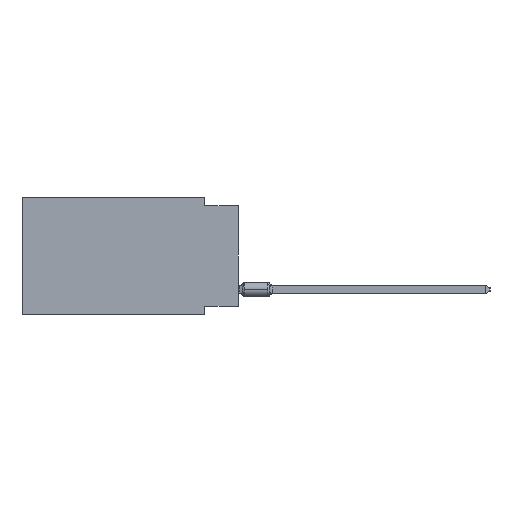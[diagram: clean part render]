
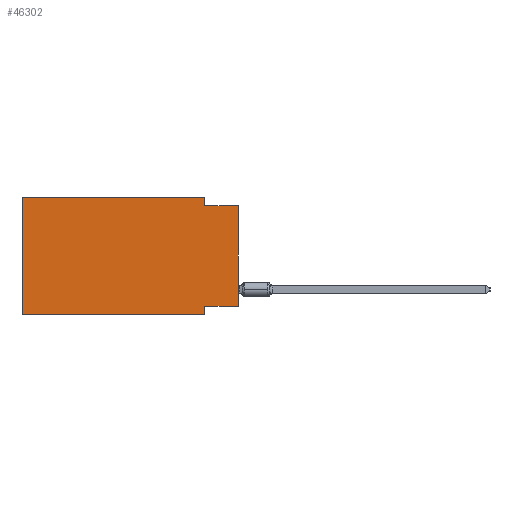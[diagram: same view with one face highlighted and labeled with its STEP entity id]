
A CAD part, left-side view. The second image highlights one B-rep face of the part: STEP entity #46302.
In plain terms, the highlighted planar face has unit normal (-1, 0, 0).
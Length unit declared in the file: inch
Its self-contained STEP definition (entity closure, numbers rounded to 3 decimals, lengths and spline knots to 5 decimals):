
#163 = DIRECTION ( 'NONE',  ( 0., -1., 0. ) ) ;
#812 = DIRECTION ( 'NONE',  ( 0., 0., -1. ) ) ;
#1198 = VECTOR ( 'NONE', #1900, 39.37008 ) ;
#1242 = ORIENTED_EDGE ( 'NONE', *, *, #15102, .F. ) ;
#1676 = ORIENTED_EDGE ( 'NONE', *, *, #29330, .T. ) ;
#1728 = DIRECTION ( 'NONE',  ( 0., -1., 0. ) ) ;
#1900 = DIRECTION ( 'NONE',  ( 0., 0., -1. ) ) ;
#2158 = LINE ( 'NONE', #32394, #14801 ) ;
#2574 = CARTESIAN_POINT ( 'NONE',  ( 0., 0., -0.025 ) ) ;
#2705 = VERTEX_POINT ( 'NONE', #45816 ) ;
#2836 = LINE ( 'NONE', #2574, #11918 ) ;
#2843 = CARTESIAN_POINT ( 'NONE',  ( 0., 0., -0.325 ) ) ;
#4345 = VERTEX_POINT ( 'NONE', #2843 ) ;
#4667 = CARTESIAN_POINT ( 'NONE',  ( 0., 0.1, 0. ) ) ;
#4724 = EDGE_CURVE ( 'NONE', #31805, #2705, #32024, .T. ) ;
#7546 = CARTESIAN_POINT ( 'NONE',  ( 0., 0., -0.025 ) ) ;
#8001 = PLANE ( 'NONE',  #42206 ) ;
#8269 = CARTESIAN_POINT ( 'NONE',  ( 0., 0.1, -0.025 ) ) ;
#8739 = CARTESIAN_POINT ( 'NONE',  ( 0., 0.645, 0. ) ) ;
#9104 = EDGE_CURVE ( 'NONE', #40372, #28077, #33290, .T. ) ;
#9225 = DIRECTION ( 'NONE',  ( 0., 0., 1. ) ) ;
#10841 = CARTESIAN_POINT ( 'NONE',  ( 0., 0.645, 0. ) ) ;
#11918 = VECTOR ( 'NONE', #13502, 39.37008 ) ;
#12370 = EDGE_CURVE ( 'NONE', #4345, #40372, #2158, .T. ) ;
#13502 = DIRECTION ( 'NONE',  ( 0., -1., 0. ) ) ;
#14061 = VECTOR ( 'NONE', #1728, 39.37008 ) ;
#14317 = LINE ( 'NONE', #35855, #1198 ) ;
#14801 = VECTOR ( 'NONE', #47782, 39.37008 ) ;
#14914 = VECTOR ( 'NONE', #24438, 39.37008 ) ;
#14999 = CARTESIAN_POINT ( 'NONE',  ( 0., 0.645, -0.35 ) ) ;
#15102 = EDGE_CURVE ( 'NONE', #2705, #39502, #34128, .T. ) ;
#15325 = VECTOR ( 'NONE', #9225, 39.37008 ) ;
#15462 = DIRECTION ( 'NONE',  ( 1., 0., 0. ) ) ;
#15937 = ORIENTED_EDGE ( 'NONE', *, *, #23910, .F. ) ;
#18026 = LINE ( 'NONE', #43304, #14914 ) ;
#18209 = VECTOR ( 'NONE', #163, 39.37008 ) ;
#20584 = LINE ( 'NONE', #35695, #14061 ) ;
#23910 = EDGE_CURVE ( 'NONE', #39502, #34939, #14317, .T. ) ;
#24438 = DIRECTION ( 'NONE',  ( 0., 0., 1. ) ) ;
#27316 = CARTESIAN_POINT ( 'NONE',  ( 0., 0.645, 0. ) ) ;
#27568 = FACE_OUTER_BOUND ( 'NONE', #31305, .T. ) ;
#28077 = VERTEX_POINT ( 'NONE', #41349 ) ;
#29242 = ORIENTED_EDGE ( 'NONE', *, *, #4724, .F. ) ;
#29330 = EDGE_CURVE ( 'NONE', #4345, #31835, #18026, .T. ) ;
#29802 = CARTESIAN_POINT ( 'NONE',  ( 0., 0.1, -0.35 ) ) ;
#30012 = CARTESIAN_POINT ( 'NONE',  ( 0., 0.1, -0.325 ) ) ;
#31305 = EDGE_LOOP ( 'NONE', ( #1676, #48799, #15937, #1242, #29242, #46632, #37430, #47811 ) ) ;
#31805 = VERTEX_POINT ( 'NONE', #14999 ) ;
#31835 = VERTEX_POINT ( 'NONE', #7546 ) ;
#32024 = LINE ( 'NONE', #8739, #15325 ) ;
#32394 = CARTESIAN_POINT ( 'NONE',  ( 0., 0., -0.325 ) ) ;
#33290 = LINE ( 'NONE', #29802, #38431 ) ;
#34128 = LINE ( 'NONE', #10841, #18209 ) ;
#34939 = VERTEX_POINT ( 'NONE', #8269 ) ;
#35695 = CARTESIAN_POINT ( 'NONE',  ( 0., 0.645, -0.35 ) ) ;
#35855 = CARTESIAN_POINT ( 'NONE',  ( 0., 0.1, 0. ) ) ;
#36416 = EDGE_CURVE ( 'NONE', #31805, #28077, #20584, .T. ) ;
#37430 = ORIENTED_EDGE ( 'NONE', *, *, #9104, .F. ) ;
#38431 = VECTOR ( 'NONE', #48437, 39.37008 ) ;
#39502 = VERTEX_POINT ( 'NONE', #4667 ) ;
#40372 = VERTEX_POINT ( 'NONE', #30012 ) ;
#41114 = EDGE_CURVE ( 'NONE', #34939, #31835, #2836, .T. ) ;
#41349 = CARTESIAN_POINT ( 'NONE',  ( 0., 0.1, -0.35 ) ) ;
#42206 = AXIS2_PLACEMENT_3D ( 'NONE', #27316, #15462, #812 ) ;
#43304 = CARTESIAN_POINT ( 'NONE',  ( 0., 0., 0. ) ) ;
#45816 = CARTESIAN_POINT ( 'NONE',  ( 0., 0.645, 0. ) ) ;
#46302 = ADVANCED_FACE ( 'NONE', ( #27568 ), #8001, .F. ) ;
#46632 = ORIENTED_EDGE ( 'NONE', *, *, #36416, .T. ) ;
#47782 = DIRECTION ( 'NONE',  ( 0., 1., 0. ) ) ;
#47811 = ORIENTED_EDGE ( 'NONE', *, *, #12370, .F. ) ;
#48437 = DIRECTION ( 'NONE',  ( 0., 0., -1. ) ) ;
#48799 = ORIENTED_EDGE ( 'NONE', *, *, #41114, .F. ) ;
